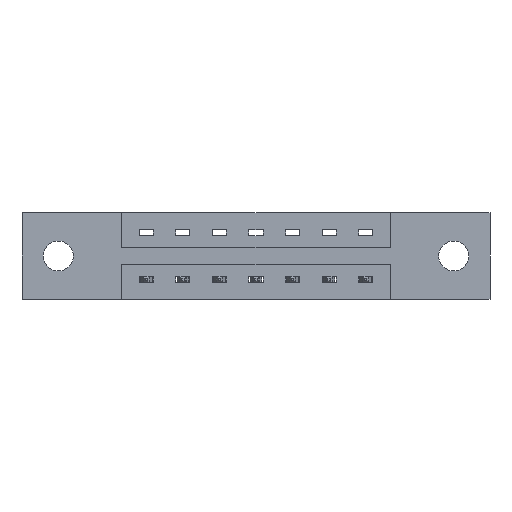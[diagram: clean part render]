
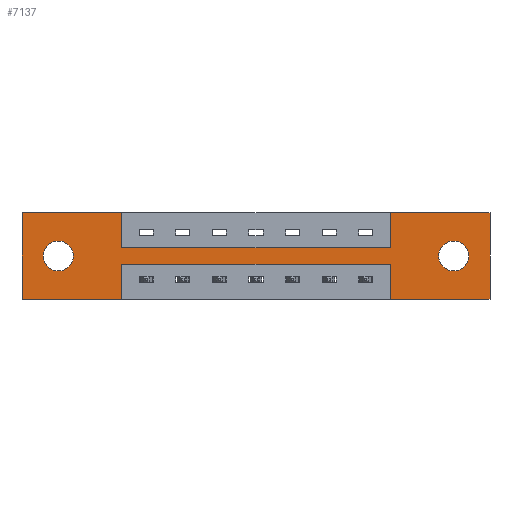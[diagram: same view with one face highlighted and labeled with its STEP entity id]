
A CAD part, front view. The second image highlights one B-rep face of the part: STEP entity #7137.
In plain terms, the highlighted planar face has unit normal (0, -1, 0).
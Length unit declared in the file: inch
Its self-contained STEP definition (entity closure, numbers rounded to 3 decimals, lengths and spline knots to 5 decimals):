
#119 = DIRECTION ( 'NONE',  ( 0., 0., -1. ) ) ;
#174 = CARTESIAN_POINT ( 'NONE',  ( 0.425, 0., -0.37 ) ) ;
#212 = EDGE_CURVE ( 'NONE', #7121, #731, #8532, .T. ) ;
#267 = VERTEX_POINT ( 'NONE', #6118 ) ;
#273 = VERTEX_POINT ( 'NONE', #6182 ) ;
#283 = DIRECTION ( 'NONE',  ( 1., 0., 0. ) ) ;
#360 = CARTESIAN_POINT ( 'NONE',  ( 0., 0., -0.37 ) ) ;
#479 = DIRECTION ( 'NONE',  ( 0., 0., 1. ) ) ;
#490 = DIRECTION ( 'NONE',  ( 0., 1., 0. ) ) ;
#505 = CARTESIAN_POINT ( 'NONE',  ( 0.155, 0., -0.185 ) ) ;
#620 = VECTOR ( 'NONE', #119, 39.37008 ) ;
#646 = DIRECTION ( 'NONE',  ( -1., 0., 0. ) ) ;
#685 = VERTEX_POINT ( 'NONE', #8382 ) ;
#731 = VERTEX_POINT ( 'NONE', #3246 ) ;
#756 = VERTEX_POINT ( 'NONE', #3763 ) ;
#1146 = AXIS2_PLACEMENT_3D ( 'NONE', #6304, #9209, #9257 ) ;
#1253 = CARTESIAN_POINT ( 'NONE',  ( 0.425, 0., -0.15 ) ) ;
#1387 = ORIENTED_EDGE ( 'NONE', *, *, #7327, .T. ) ;
#1397 = CARTESIAN_POINT ( 'NONE',  ( 1.843, 0., -0.185 ) ) ;
#1455 = LINE ( 'NONE', #4788, #9172 ) ;
#1496 = VERTEX_POINT ( 'NONE', #4957 ) ;
#1588 = CARTESIAN_POINT ( 'NONE',  ( 0.425, 0., -0.15 ) ) ;
#1705 = EDGE_CURVE ( 'NONE', #3506, #5985, #6650, .T. ) ;
#1732 = ORIENTED_EDGE ( 'NONE', *, *, #4045, .T. ) ;
#1823 = ORIENTED_EDGE ( 'NONE', *, *, #4613, .T. ) ;
#1903 = LINE ( 'NONE', #3096, #9524 ) ;
#2003 = ORIENTED_EDGE ( 'NONE', *, *, #6317, .T. ) ;
#2051 = DIRECTION ( 'NONE',  ( 0., 0., 1. ) ) ;
#2148 = ORIENTED_EDGE ( 'NONE', *, *, #1705, .F. ) ;
#2166 = CARTESIAN_POINT ( 'NONE',  ( 0.155, 0., -0.121 ) ) ;
#2173 = CIRCLE ( 'NONE', #3323, 0.064 ) ;
#2208 = DIRECTION ( 'NONE',  ( 0., 0., -1. ) ) ;
#2212 = DIRECTION ( 'NONE',  ( 0., 1., 0. ) ) ;
#2271 = LINE ( 'NONE', #4006, #6134 ) ;
#2298 = ORIENTED_EDGE ( 'NONE', *, *, #8002, .F. ) ;
#2348 = ORIENTED_EDGE ( 'NONE', *, *, #212, .F. ) ;
#2388 = FACE_BOUND ( 'NONE', #9671, .T. ) ;
#2398 = DIRECTION ( 'NONE',  ( 0., 0., -1. ) ) ;
#2485 = ORIENTED_EDGE ( 'NONE', *, *, #7674, .F. ) ;
#2557 = CIRCLE ( 'NONE', #7426, 0.064 ) ;
#2590 = ORIENTED_EDGE ( 'NONE', *, *, #7941, .F. ) ;
#2737 = ORIENTED_EDGE ( 'NONE', *, *, #3066, .F. ) ;
#2778 = VECTOR ( 'NONE', #2398, 39.37008 ) ;
#2811 = VECTOR ( 'NONE', #9169, 39.37008 ) ;
#2902 = CARTESIAN_POINT ( 'NONE',  ( 1.573, 0., 0. ) ) ;
#2923 = CARTESIAN_POINT ( 'NONE',  ( 1.573, 0., -0.15 ) ) ;
#3066 = EDGE_CURVE ( 'NONE', #4529, #685, #2271, .T. ) ;
#3096 = CARTESIAN_POINT ( 'NONE',  ( 0., 0., -0.37 ) ) ;
#3177 = VECTOR ( 'NONE', #283, 39.37008 ) ;
#3186 = CARTESIAN_POINT ( 'NONE',  ( 0.425, 0., -0.37 ) ) ;
#3246 = CARTESIAN_POINT ( 'NONE',  ( 1.573, 0., -0.22 ) ) ;
#3323 = AXIS2_PLACEMENT_3D ( 'NONE', #505, #490, #479 ) ;
#3420 = LINE ( 'NONE', #7349, #3177 ) ;
#3423 = CARTESIAN_POINT ( 'NONE',  ( 0.425, 0., 0. ) ) ;
#3452 = LINE ( 'NONE', #5454, #9108 ) ;
#3506 = VERTEX_POINT ( 'NONE', #8598 ) ;
#3763 = CARTESIAN_POINT ( 'NONE',  ( 1.998, 0., -0.37 ) ) ;
#3828 = CARTESIAN_POINT ( 'NONE',  ( 0., 0., 0. ) ) ;
#3917 = EDGE_CURVE ( 'NONE', #267, #8001, #1455, .T. ) ;
#3955 = AXIS2_PLACEMENT_3D ( 'NONE', #4999, #6488, #6669 ) ;
#4006 = CARTESIAN_POINT ( 'NONE',  ( 0., 0., 0. ) ) ;
#4045 = EDGE_CURVE ( 'NONE', #1496, #8350, #2557, .T. ) ;
#4391 = ORIENTED_EDGE ( 'NONE', *, *, #9244, .F. ) ;
#4413 = LINE ( 'NONE', #6407, #6224 ) ;
#4529 = VERTEX_POINT ( 'NONE', #8440 ) ;
#4613 = EDGE_CURVE ( 'NONE', #6227, #273, #9264, .T. ) ;
#4788 = CARTESIAN_POINT ( 'NONE',  ( 0., 0., 0. ) ) ;
#4908 = VECTOR ( 'NONE', #5293, 39.37008 ) ;
#4957 = CARTESIAN_POINT ( 'NONE',  ( 1.843, 0., -0.249 ) ) ;
#4970 = VERTEX_POINT ( 'NONE', #9029 ) ;
#4999 = CARTESIAN_POINT ( 'NONE',  ( 0.155, 0., -0.185 ) ) ;
#5043 = LINE ( 'NONE', #360, #6848 ) ;
#5053 = CIRCLE ( 'NONE', #7383, 0.064 ) ;
#5293 = DIRECTION ( 'NONE',  ( 1., 0., 0. ) ) ;
#5297 = VERTEX_POINT ( 'NONE', #2923 ) ;
#5363 = DIRECTION ( 'NONE',  ( -1., 0., 0. ) ) ;
#5454 = CARTESIAN_POINT ( 'NONE',  ( 0.425, 0., -0.22 ) ) ;
#5985 = VERTEX_POINT ( 'NONE', #3186 ) ;
#6045 = EDGE_CURVE ( 'NONE', #4970, #6322, #7112, .T. ) ;
#6104 = EDGE_CURVE ( 'NONE', #5297, #4529, #8267, .T. ) ;
#6118 = CARTESIAN_POINT ( 'NONE',  ( 0., 0., -0.37 ) ) ;
#6134 = VECTOR ( 'NONE', #7746, 39.37008 ) ;
#6182 = CARTESIAN_POINT ( 'NONE',  ( 0.155, 0., -0.249 ) ) ;
#6224 = VECTOR ( 'NONE', #9461, 39.37008 ) ;
#6227 = VERTEX_POINT ( 'NONE', #2166 ) ;
#6261 = DIRECTION ( 'NONE',  ( -1., 0., 0. ) ) ;
#6304 = CARTESIAN_POINT ( 'NONE',  ( 0., 0., -0.37 ) ) ;
#6317 = EDGE_CURVE ( 'NONE', #273, #6227, #2173, .T. ) ;
#6322 = VERTEX_POINT ( 'NONE', #1588 ) ;
#6392 = VECTOR ( 'NONE', #2051, 39.37008 ) ;
#6407 = CARTESIAN_POINT ( 'NONE',  ( 1.998, 0., 0. ) ) ;
#6488 = DIRECTION ( 'NONE',  ( 0., 1., 0. ) ) ;
#6650 = LINE ( 'NONE', #174, #620 ) ;
#6656 = CARTESIAN_POINT ( 'NONE',  ( 1.573, 0., -0.37 ) ) ;
#6669 = DIRECTION ( 'NONE',  ( 0., 0., 1. ) ) ;
#6728 = FACE_OUTER_BOUND ( 'NONE', #6770, .T. ) ;
#6770 = EDGE_LOOP ( 'NONE', ( #2148, #2298, #2348, #2485, #2590, #2737, #7823, #7812, #7352, #4391, #6826, #9156 ) ) ;
#6826 = ORIENTED_EDGE ( 'NONE', *, *, #3917, .F. ) ;
#6848 = VECTOR ( 'NONE', #646, 39.37008 ) ;
#6897 = DIRECTION ( 'NONE',  ( 0., 0., 1. ) ) ;
#7112 = LINE ( 'NONE', #3423, #2778 ) ;
#7121 = VERTEX_POINT ( 'NONE', #6656 ) ;
#7137 = ADVANCED_FACE ( 'NONE', ( #8150, #2388, #6728 ), #9647, .T. ) ;
#7327 = EDGE_CURVE ( 'NONE', #8350, #1496, #5053, .T. ) ;
#7349 = CARTESIAN_POINT ( 'NONE',  ( 0., 0., 0. ) ) ;
#7352 = ORIENTED_EDGE ( 'NONE', *, *, #6045, .F. ) ;
#7383 = AXIS2_PLACEMENT_3D ( 'NONE', #9389, #9359, #9339 ) ;
#7426 = AXIS2_PLACEMENT_3D ( 'NONE', #1397, #2212, #2208 ) ;
#7490 = EDGE_LOOP ( 'NONE', ( #1387, #1732 ) ) ;
#7674 = EDGE_CURVE ( 'NONE', #756, #7121, #5043, .T. ) ;
#7746 = DIRECTION ( 'NONE',  ( 1., 0., 0. ) ) ;
#7812 = ORIENTED_EDGE ( 'NONE', *, *, #8244, .F. ) ;
#7823 = ORIENTED_EDGE ( 'NONE', *, *, #6104, .F. ) ;
#7941 = EDGE_CURVE ( 'NONE', #685, #756, #4413, .T. ) ;
#8001 = VERTEX_POINT ( 'NONE', #3828 ) ;
#8002 = EDGE_CURVE ( 'NONE', #731, #3506, #3452, .T. ) ;
#8150 = FACE_BOUND ( 'NONE', #7490, .T. ) ;
#8244 = EDGE_CURVE ( 'NONE', #6322, #5297, #8765, .T. ) ;
#8267 = LINE ( 'NONE', #2902, #6392 ) ;
#8330 = EDGE_CURVE ( 'NONE', #5985, #267, #1903, .T. ) ;
#8350 = VERTEX_POINT ( 'NONE', #9235 ) ;
#8382 = CARTESIAN_POINT ( 'NONE',  ( 1.998, 0., 0. ) ) ;
#8440 = CARTESIAN_POINT ( 'NONE',  ( 1.573, 0., 0. ) ) ;
#8532 = LINE ( 'NONE', #9611, #2811 ) ;
#8598 = CARTESIAN_POINT ( 'NONE',  ( 0.425, 0., -0.22 ) ) ;
#8765 = LINE ( 'NONE', #1253, #4908 ) ;
#9029 = CARTESIAN_POINT ( 'NONE',  ( 0.425, 0., 0. ) ) ;
#9108 = VECTOR ( 'NONE', #6261, 39.37008 ) ;
#9156 = ORIENTED_EDGE ( 'NONE', *, *, #8330, .F. ) ;
#9169 = DIRECTION ( 'NONE',  ( 0., 0., 1. ) ) ;
#9172 = VECTOR ( 'NONE', #6897, 39.37008 ) ;
#9209 = DIRECTION ( 'NONE',  ( 0., -1., 0. ) ) ;
#9235 = CARTESIAN_POINT ( 'NONE',  ( 1.843, 0., -0.121 ) ) ;
#9244 = EDGE_CURVE ( 'NONE', #8001, #4970, #3420, .T. ) ;
#9257 = DIRECTION ( 'NONE',  ( 0., 0., -1. ) ) ;
#9264 = CIRCLE ( 'NONE', #3955, 0.064 ) ;
#9339 = DIRECTION ( 'NONE',  ( 0., 0., -1. ) ) ;
#9359 = DIRECTION ( 'NONE',  ( 0., 1., 0. ) ) ;
#9389 = CARTESIAN_POINT ( 'NONE',  ( 1.843, 0., -0.185 ) ) ;
#9461 = DIRECTION ( 'NONE',  ( 0., 0., -1. ) ) ;
#9524 = VECTOR ( 'NONE', #5363, 39.37008 ) ;
#9611 = CARTESIAN_POINT ( 'NONE',  ( 1.573, 0., -0.37 ) ) ;
#9647 = PLANE ( 'NONE',  #1146 ) ;
#9671 = EDGE_LOOP ( 'NONE', ( #1823, #2003 ) ) ;
